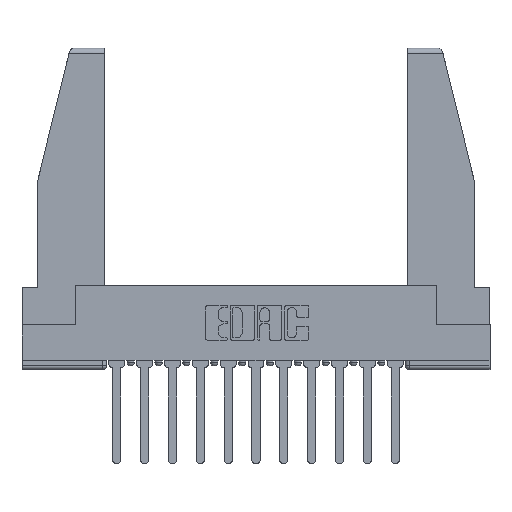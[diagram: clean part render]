
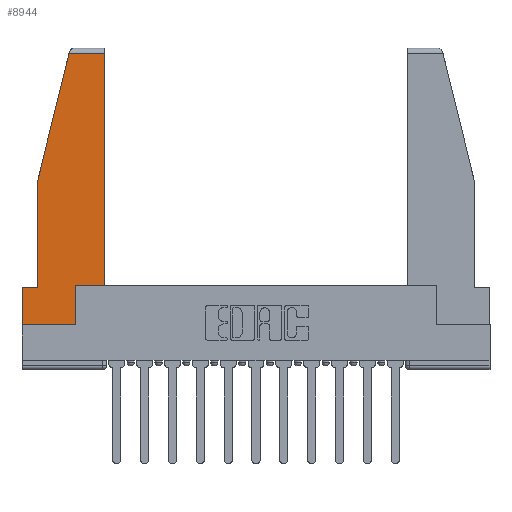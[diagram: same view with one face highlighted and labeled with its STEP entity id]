
A CAD part, top view. The second image highlights one B-rep face of the part: STEP entity #8944.
In plain terms, the highlighted planar face has unit normal (0, 0, 1).
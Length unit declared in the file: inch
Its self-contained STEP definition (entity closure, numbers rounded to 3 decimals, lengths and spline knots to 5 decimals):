
#16 = CARTESIAN_POINT ( 'NONE',  ( 0.271, 1.55, 0. ) ) ;
#421 = CARTESIAN_POINT ( 'NONE',  ( 0.086, 0.21, 0. ) ) ;
#579 = ORIENTED_EDGE ( 'NONE', *, *, #1128, .T. ) ;
#774 = EDGE_CURVE ( 'NONE', #9931, #15019, #3859, .T. ) ;
#978 = PLANE ( 'NONE',  #11885 ) ;
#1054 = CARTESIAN_POINT ( 'NONE',  ( 0., 0., 0. ) ) ;
#1101 = DIRECTION ( 'NONE',  ( -1., 0., 0. ) ) ;
#1128 = EDGE_CURVE ( 'NONE', #10201, #9931, #15843, .T. ) ;
#1149 = VECTOR ( 'NONE', #14321, 39.37008 ) ;
#1425 = CARTESIAN_POINT ( 'NONE',  ( 0., 0.21, 0. ) ) ;
#1470 = VERTEX_POINT ( 'NONE', #8117 ) ;
#1730 = VECTOR ( 'NONE', #7898, 39.37008 ) ;
#1939 = VECTOR ( 'NONE', #6370, 39.37008 ) ;
#2067 = CARTESIAN_POINT ( 'NONE',  ( 0.086, 0.8, 0. ) ) ;
#2122 = CARTESIAN_POINT ( 'NONE',  ( 0., 0., 0. ) ) ;
#2252 = ORIENTED_EDGE ( 'NONE', *, *, #10818, .T. ) ;
#2260 = DIRECTION ( 'NONE',  ( 0., 1., 0. ) ) ;
#2276 = ORIENTED_EDGE ( 'NONE', *, *, #6216, .T. ) ;
#3020 = EDGE_CURVE ( 'NONE', #15019, #9661, #10993, .T. ) ;
#3337 = VECTOR ( 'NONE', #7081, 39.37008 ) ;
#3393 = EDGE_CURVE ( 'NONE', #13638, #13452, #9364, .T. ) ;
#3850 = VECTOR ( 'NONE', #2260, 39.37008 ) ;
#3859 = LINE ( 'NONE', #7445, #1939 ) ;
#3981 = CARTESIAN_POINT ( 'NONE',  ( 0.461, 1.52, 0. ) ) ;
#4055 = VERTEX_POINT ( 'NONE', #14261 ) ;
#4308 = EDGE_LOOP ( 'NONE', ( #2252, #11190, #579, #6067, #12253, #2276, #11825, #8508, #5057 ) ) ;
#4945 = DIRECTION ( 'NONE',  ( -0.239, -0.971, 0. ) ) ;
#5057 = ORIENTED_EDGE ( 'NONE', *, *, #3393, .T. ) ;
#5146 = CARTESIAN_POINT ( 'NONE',  ( 0.461, 0.223, 0. ) ) ;
#6067 = ORIENTED_EDGE ( 'NONE', *, *, #774, .T. ) ;
#6216 = EDGE_CURVE ( 'NONE', #9661, #1470, #13908, .T. ) ;
#6370 = DIRECTION ( 'NONE',  ( 0., -1., 0. ) ) ;
#7062 = LINE ( 'NONE', #15824, #3850 ) ;
#7081 = DIRECTION ( 'NONE',  ( 1., 0., 0. ) ) ;
#7321 = EDGE_CURVE ( 'NONE', #1470, #4055, #13154, .T. ) ;
#7421 = VERTEX_POINT ( 'NONE', #3981 ) ;
#7445 = CARTESIAN_POINT ( 'NONE',  ( 0.086, 0.8, 0. ) ) ;
#7583 = EDGE_CURVE ( 'NONE', #4055, #13638, #7062, .T. ) ;
#7898 = DIRECTION ( 'NONE',  ( 0., -1., 0. ) ) ;
#8117 = CARTESIAN_POINT ( 'NONE',  ( 0., 0., 0. ) ) ;
#8437 = DIRECTION ( 'NONE',  ( 1., 0., 0. ) ) ;
#8508 = ORIENTED_EDGE ( 'NONE', *, *, #7583, .T. ) ;
#8944 = ADVANCED_FACE ( 'NONE', ( #12083 ), #978, .T. ) ;
#9317 = VECTOR ( 'NONE', #14939, 39.37008 ) ;
#9364 = LINE ( 'NONE', #11875, #1149 ) ;
#9653 = DIRECTION ( 'NONE',  ( 0., 0., 1. ) ) ;
#9661 = VERTEX_POINT ( 'NONE', #1425 ) ;
#9702 = VECTOR ( 'NONE', #1101, 39.37008 ) ;
#9887 = CARTESIAN_POINT ( 'NONE',  ( 0., 1.52, 0. ) ) ;
#9931 = VERTEX_POINT ( 'NONE', #2067 ) ;
#9970 = LINE ( 'NONE', #9887, #9317 ) ;
#10111 = LINE ( 'NONE', #13609, #12423 ) ;
#10201 = VERTEX_POINT ( 'NONE', #11466 ) ;
#10818 = EDGE_CURVE ( 'NONE', #13452, #7421, #10111, .T. ) ;
#10993 = LINE ( 'NONE', #14910, #9702 ) ;
#11163 = DIRECTION ( 'NONE',  ( 0., 1., 0. ) ) ;
#11190 = ORIENTED_EDGE ( 'NONE', *, *, #11309, .T. ) ;
#11309 = EDGE_CURVE ( 'NONE', #7421, #10201, #9970, .T. ) ;
#11466 = CARTESIAN_POINT ( 'NONE',  ( 0.2636, 1.52, 0. ) ) ;
#11542 = CARTESIAN_POINT ( 'NONE',  ( 0., 0.21, 0. ) ) ;
#11825 = ORIENTED_EDGE ( 'NONE', *, *, #7321, .T. ) ;
#11875 = CARTESIAN_POINT ( 'NONE',  ( 0.297, 0.223, 0. ) ) ;
#11885 = AXIS2_PLACEMENT_3D ( 'NONE', #1054, #9653, #8437 ) ;
#12039 = VECTOR ( 'NONE', #4945, 39.37008 ) ;
#12083 = FACE_OUTER_BOUND ( 'NONE', #4308, .T. ) ;
#12253 = ORIENTED_EDGE ( 'NONE', *, *, #3020, .T. ) ;
#12423 = VECTOR ( 'NONE', #11163, 39.37008 ) ;
#13154 = LINE ( 'NONE', #2122, #3337 ) ;
#13452 = VERTEX_POINT ( 'NONE', #5146 ) ;
#13609 = CARTESIAN_POINT ( 'NONE',  ( 0.461, 0.223, 0. ) ) ;
#13638 = VERTEX_POINT ( 'NONE', #14153 ) ;
#13908 = LINE ( 'NONE', #11542, #1730 ) ;
#14153 = CARTESIAN_POINT ( 'NONE',  ( 0.297, 0.223, 0. ) ) ;
#14261 = CARTESIAN_POINT ( 'NONE',  ( 0.297, 0., 0. ) ) ;
#14321 = DIRECTION ( 'NONE',  ( 1., 0., 0. ) ) ;
#14910 = CARTESIAN_POINT ( 'NONE',  ( 0., 0.21, 0. ) ) ;
#14939 = DIRECTION ( 'NONE',  ( -1., 0., 0. ) ) ;
#15019 = VERTEX_POINT ( 'NONE', #421 ) ;
#15824 = CARTESIAN_POINT ( 'NONE',  ( 0.297, 0., 0. ) ) ;
#15843 = LINE ( 'NONE', #16, #12039 ) ;
